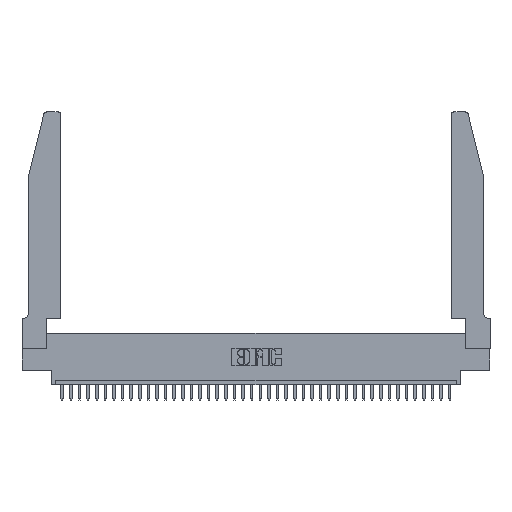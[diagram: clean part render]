
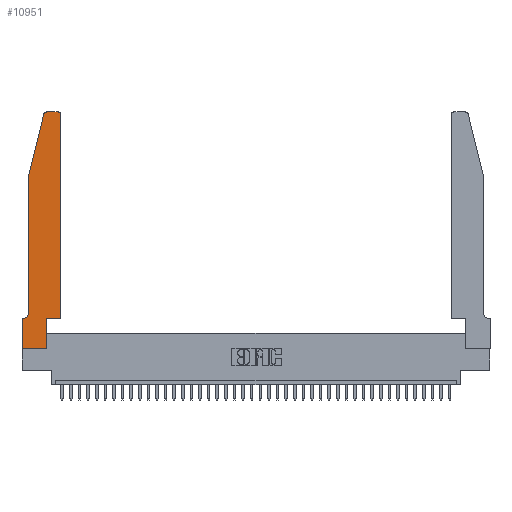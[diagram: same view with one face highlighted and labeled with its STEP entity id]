
A CAD part, top view. The second image highlights one B-rep face of the part: STEP entity #10951.
In plain terms, the highlighted planar face has unit normal (0, 0, 1).
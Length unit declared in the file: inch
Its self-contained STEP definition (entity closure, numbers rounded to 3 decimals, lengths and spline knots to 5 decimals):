
#510 = CARTESIAN_POINT ( 'NONE',  ( 0.0055, 0.42, 0.37 ) ) ;
#913 = CIRCLE ( 'NONE', #22025, 0.03 ) ;
#1064 = DIRECTION ( 'NONE',  ( -1., 0., 0. ) ) ;
#1075 = CARTESIAN_POINT ( 'NONE',  ( 0., 0., 0.37 ) ) ;
#1171 = EDGE_CURVE ( 'NONE', #12787, #20936, #15508, .T. ) ;
#1291 = ORIENTED_EDGE ( 'NONE', *, *, #4550, .T. ) ;
#2059 = DIRECTION ( 'NONE',  ( 0., 0., 1. ) ) ;
#2076 = LINE ( 'NONE', #22565, #8699 ) ;
#2533 = VERTEX_POINT ( 'NONE', #25209 ) ;
#2852 = ORIENTED_EDGE ( 'NONE', *, *, #13612, .T. ) ;
#2946 = CARTESIAN_POINT ( 'NONE',  ( 0.284, 2.75, 0.37 ) ) ;
#2974 = CARTESIAN_POINT ( 'NONE',  ( 0.0755, 2., 0.37 ) ) ;
#3053 = VECTOR ( 'NONE', #25997, 39.37008 ) ;
#3458 = EDGE_LOOP ( 'NONE', ( #4940, #30132, #2852, #1291, #4547, #31049, #37959, #38422, #9571, #34906, #14846, #22082 ) ) ;
#3877 = DIRECTION ( 'NONE',  ( 0., 0., 1. ) ) ;
#3968 = EDGE_CURVE ( 'NONE', #2533, #12787, #24504, .T. ) ;
#4016 = DIRECTION ( 'NONE',  ( 1., 0., 0. ) ) ;
#4169 = EDGE_CURVE ( 'NONE', #14734, #19095, #913, .T. ) ;
#4227 = VECTOR ( 'NONE', #20290, 39.37008 ) ;
#4547 = ORIENTED_EDGE ( 'NONE', *, *, #27227, .T. ) ;
#4550 = EDGE_CURVE ( 'NONE', #34872, #11502, #12242, .T. ) ;
#4940 = ORIENTED_EDGE ( 'NONE', *, *, #21986, .T. ) ;
#5151 = CARTESIAN_POINT ( 'NONE',  ( 0., 0.35, 0.37 ) ) ;
#6266 = CARTESIAN_POINT ( 'NONE',  ( 0.4205, 2.75, 0.37 ) ) ;
#6636 = CARTESIAN_POINT ( 'NONE',  ( 0.4205, 2.72, 0.37 ) ) ;
#7634 = DIRECTION ( 'NONE',  ( -0.239, -0.971, 0. ) ) ;
#8098 = VECTOR ( 'NONE', #23621, 39.37008 ) ;
#8699 = VECTOR ( 'NONE', #7634, 39.37008 ) ;
#9571 = ORIENTED_EDGE ( 'NONE', *, *, #24122, .T. ) ;
#9903 = DIRECTION ( 'NONE',  ( 0., 0., -1. ) ) ;
#10951 = ADVANCED_FACE ( 'NONE', ( #26320 ), #23927, .T. ) ;
#10986 = CARTESIAN_POINT ( 'NONE',  ( 0.2865, 0., 0.37 ) ) ;
#11237 = CARTESIAN_POINT ( 'NONE',  ( 0.2865, 0.35, 0.37 ) ) ;
#11502 = VERTEX_POINT ( 'NONE', #15958 ) ;
#11861 = DIRECTION ( 'NONE',  ( 1., 0., 0. ) ) ;
#11941 = CARTESIAN_POINT ( 'NONE',  ( 0.0755, 0.35, 0.37 ) ) ;
#12242 = LINE ( 'NONE', #2974, #32598 ) ;
#12452 = VERTEX_POINT ( 'NONE', #25099 ) ;
#12787 = VERTEX_POINT ( 'NONE', #34610 ) ;
#13060 = DIRECTION ( 'NONE',  ( 0., -1., 0. ) ) ;
#13418 = VECTOR ( 'NONE', #36129, 39.37008 ) ;
#13612 = EDGE_CURVE ( 'NONE', #19095, #34872, #2076, .T. ) ;
#14003 = EDGE_CURVE ( 'NONE', #20936, #23590, #20962, .T. ) ;
#14184 = CARTESIAN_POINT ( 'NONE',  ( 0.4505, 0.35, 0.37 ) ) ;
#14186 = AXIS2_PLACEMENT_3D ( 'NONE', #6636, #3877, #4016 ) ;
#14242 = CARTESIAN_POINT ( 'NONE',  ( 0., 0., 0.37 ) ) ;
#14734 = VERTEX_POINT ( 'NONE', #2946 ) ;
#14846 = ORIENTED_EDGE ( 'NONE', *, *, #1171, .T. ) ;
#15508 = LINE ( 'NONE', #14184, #24496 ) ;
#15797 = LINE ( 'NONE', #11237, #3053 ) ;
#15958 = CARTESIAN_POINT ( 'NONE',  ( 0.0755, 0.42, 0.37 ) ) ;
#16089 = LINE ( 'NONE', #37934, #4227 ) ;
#16468 = VECTOR ( 'NONE', #13060, 39.37008 ) ;
#18175 = AXIS2_PLACEMENT_3D ( 'NONE', #26041, #2059, #23181 ) ;
#18607 = VERTEX_POINT ( 'NONE', #10986 ) ;
#19095 = VERTEX_POINT ( 'NONE', #37896 ) ;
#19457 = CARTESIAN_POINT ( 'NONE',  ( 0.0755, 2., 0.37 ) ) ;
#19806 = CIRCLE ( 'NONE', #20237, 0.07 ) ;
#20237 = AXIS2_PLACEMENT_3D ( 'NONE', #510, #9903, #1064 ) ;
#20290 = DIRECTION ( 'NONE',  ( -1., 0., 0. ) ) ;
#20936 = VERTEX_POINT ( 'NONE', #26278 ) ;
#20962 = CIRCLE ( 'NONE', #14186, 0.03 ) ;
#21333 = LINE ( 'NONE', #14242, #8098 ) ;
#21986 = EDGE_CURVE ( 'NONE', #23590, #14734, #16089, .T. ) ;
#22025 = AXIS2_PLACEMENT_3D ( 'NONE', #23914, #26522, #11861 ) ;
#22082 = ORIENTED_EDGE ( 'NONE', *, *, #14003, .T. ) ;
#22565 = CARTESIAN_POINT ( 'NONE',  ( 0.0755, 2., 0.37 ) ) ;
#22634 = CARTESIAN_POINT ( 'NONE',  ( 0.4505, 0.35, 0.37 ) ) ;
#22906 = DIRECTION ( 'NONE',  ( 0., 1., 0. ) ) ;
#23181 = DIRECTION ( 'NONE',  ( 1., 0., 0. ) ) ;
#23590 = VERTEX_POINT ( 'NONE', #6266 ) ;
#23621 = DIRECTION ( 'NONE',  ( 1., 0., 0. ) ) ;
#23914 = CARTESIAN_POINT ( 'NONE',  ( 0.284, 2.72, 0.37 ) ) ;
#23927 = PLANE ( 'NONE',  #18175 ) ;
#24005 = DIRECTION ( 'NONE',  ( 0., -1., 0. ) ) ;
#24122 = EDGE_CURVE ( 'NONE', #18607, #2533, #15797, .T. ) ;
#24496 = VECTOR ( 'NONE', #22906, 39.37008 ) ;
#24504 = LINE ( 'NONE', #22634, #31608 ) ;
#25099 = CARTESIAN_POINT ( 'NONE',  ( 0.0055, 0.35, 0.37 ) ) ;
#25209 = CARTESIAN_POINT ( 'NONE',  ( 0.2865, 0.35, 0.37 ) ) ;
#25997 = DIRECTION ( 'NONE',  ( 0., 1., 0. ) ) ;
#26041 = CARTESIAN_POINT ( 'NONE',  ( 0., 0.35, 0.37 ) ) ;
#26278 = CARTESIAN_POINT ( 'NONE',  ( 0.4505, 2.72, 0.37 ) ) ;
#26320 = FACE_OUTER_BOUND ( 'NONE', #3458, .T. ) ;
#26434 = DIRECTION ( 'NONE',  ( 1., 0., 0. ) ) ;
#26522 = DIRECTION ( 'NONE',  ( 0., 0., 1. ) ) ;
#27227 = EDGE_CURVE ( 'NONE', #11502, #12452, #19806, .T. ) ;
#27654 = VERTEX_POINT ( 'NONE', #35023 ) ;
#30132 = ORIENTED_EDGE ( 'NONE', *, *, #4169, .T. ) ;
#31049 = ORIENTED_EDGE ( 'NONE', *, *, #32272, .T. ) ;
#31608 = VECTOR ( 'NONE', #26434, 39.37008 ) ;
#32272 = EDGE_CURVE ( 'NONE', #12452, #35053, #33688, .T. ) ;
#32598 = VECTOR ( 'NONE', #24005, 39.37008 ) ;
#33446 = LINE ( 'NONE', #1075, #16468 ) ;
#33688 = LINE ( 'NONE', #11941, #13418 ) ;
#34610 = CARTESIAN_POINT ( 'NONE',  ( 0.4505, 0.35, 0.37 ) ) ;
#34872 = VERTEX_POINT ( 'NONE', #19457 ) ;
#34906 = ORIENTED_EDGE ( 'NONE', *, *, #3968, .T. ) ;
#35023 = CARTESIAN_POINT ( 'NONE',  ( 0., 0., 0.37 ) ) ;
#35053 = VERTEX_POINT ( 'NONE', #5151 ) ;
#35260 = EDGE_CURVE ( 'NONE', #35053, #27654, #33446, .T. ) ;
#35659 = EDGE_CURVE ( 'NONE', #27654, #18607, #21333, .T. ) ;
#36129 = DIRECTION ( 'NONE',  ( -1., 0., 0. ) ) ;
#37896 = CARTESIAN_POINT ( 'NONE',  ( 0.25487, 2.72718, 0.37 ) ) ;
#37934 = CARTESIAN_POINT ( 'NONE',  ( 0.2605, 2.75, 0.37 ) ) ;
#37959 = ORIENTED_EDGE ( 'NONE', *, *, #35260, .T. ) ;
#38422 = ORIENTED_EDGE ( 'NONE', *, *, #35659, .T. ) ;
